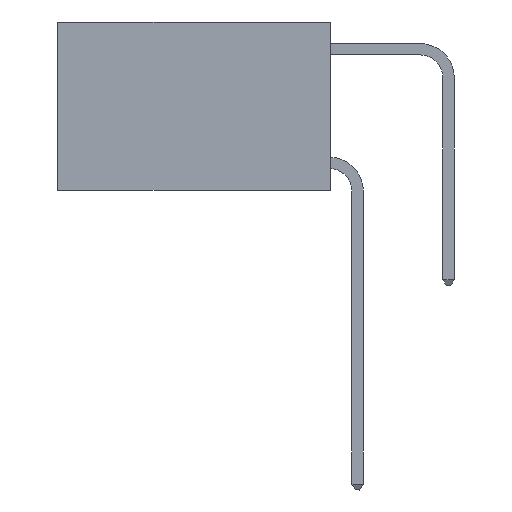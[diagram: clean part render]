
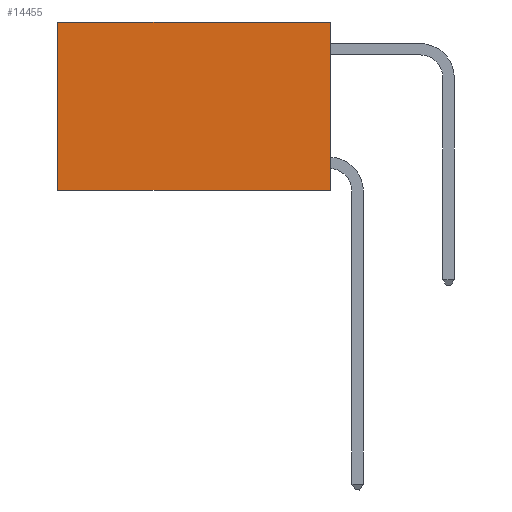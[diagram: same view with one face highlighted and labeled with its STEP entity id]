
A CAD part, left-side view. The second image highlights one B-rep face of the part: STEP entity #14455.
In plain terms, the highlighted planar face has unit normal (-1, 0, 0).
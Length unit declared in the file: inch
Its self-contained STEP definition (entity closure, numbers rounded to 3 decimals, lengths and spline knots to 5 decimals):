
#421 = ORIENTED_EDGE ( 'NONE', *, *, #10940, .T. ) ;
#1004 = PLANE ( 'NONE',  #15366 ) ;
#3111 = VECTOR ( 'NONE', #11617, 39.37008 ) ;
#3769 = DIRECTION ( 'NONE',  ( 0., 0., -1. ) ) ;
#4037 = CARTESIAN_POINT ( 'NONE',  ( 0.2625, 0., -0.37 ) ) ;
#4043 = CARTESIAN_POINT ( 'NONE',  ( 0.2625, 0., 0. ) ) ;
#4269 = CARTESIAN_POINT ( 'NONE',  ( 0.2625, 0., 0. ) ) ;
#4402 = ORIENTED_EDGE ( 'NONE', *, *, #13122, .T. ) ;
#5369 = CARTESIAN_POINT ( 'NONE',  ( 0.2625, 0., -0.37 ) ) ;
#5506 = DIRECTION ( 'NONE',  ( 0., 0., -1. ) ) ;
#5775 = VECTOR ( 'NONE', #3769, 39.37008 ) ;
#5855 = CARTESIAN_POINT ( 'NONE',  ( 0.2625, 0., 0. ) ) ;
#6082 = VECTOR ( 'NONE', #14702, 39.37008 ) ;
#6147 = VERTEX_POINT ( 'NONE', #5369 ) ;
#7909 = FACE_OUTER_BOUND ( 'NONE', #10865, .T. ) ;
#8443 = VERTEX_POINT ( 'NONE', #15083 ) ;
#8566 = VERTEX_POINT ( 'NONE', #18223 ) ;
#10865 = EDGE_LOOP ( 'NONE', ( #4402, #11671, #17680, #421 ) ) ;
#10892 = EDGE_CURVE ( 'NONE', #8443, #6147, #18688, .T. ) ;
#10940 = EDGE_CURVE ( 'NONE', #8443, #13160, #17783, .T. ) ;
#11617 = DIRECTION ( 'NONE',  ( 0., 0., -1. ) ) ;
#11671 = ORIENTED_EDGE ( 'NONE', *, *, #17214, .F. ) ;
#13122 = EDGE_CURVE ( 'NONE', #13160, #8566, #13636, .T. ) ;
#13160 = VERTEX_POINT ( 'NONE', #18478 ) ;
#13636 = LINE ( 'NONE', #15527, #5775 ) ;
#14072 = VECTOR ( 'NONE', #17242, 39.37008 ) ;
#14353 = DIRECTION ( 'NONE',  ( 1., 0., 0. ) ) ;
#14455 = ADVANCED_FACE ( 'NONE', ( #7909 ), #1004, .F. ) ;
#14702 = DIRECTION ( 'NONE',  ( 0., 1., 0. ) ) ;
#15083 = CARTESIAN_POINT ( 'NONE',  ( 0.2625, 0., 0. ) ) ;
#15366 = AXIS2_PLACEMENT_3D ( 'NONE', #4043, #14353, #5506 ) ;
#15527 = CARTESIAN_POINT ( 'NONE',  ( 0.2625, 0.6, 0. ) ) ;
#17214 = EDGE_CURVE ( 'NONE', #6147, #8566, #17918, .T. ) ;
#17242 = DIRECTION ( 'NONE',  ( 0., 1., 0. ) ) ;
#17680 = ORIENTED_EDGE ( 'NONE', *, *, #10892, .F. ) ;
#17783 = LINE ( 'NONE', #5855, #6082 ) ;
#17918 = LINE ( 'NONE', #4037, #14072 ) ;
#18223 = CARTESIAN_POINT ( 'NONE',  ( 0.2625, 0.6, -0.37 ) ) ;
#18478 = CARTESIAN_POINT ( 'NONE',  ( 0.2625, 0.6, 0. ) ) ;
#18688 = LINE ( 'NONE', #4269, #3111 ) ;
